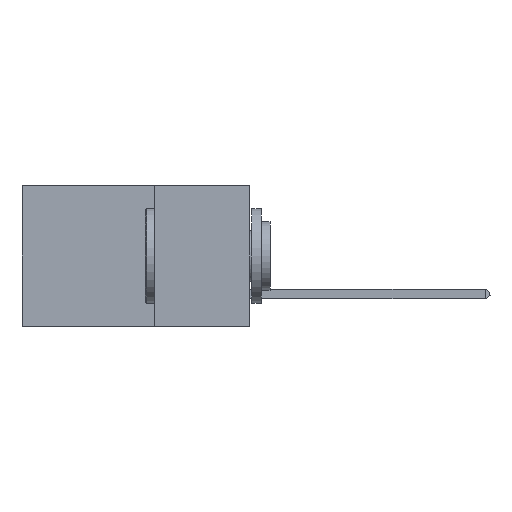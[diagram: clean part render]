
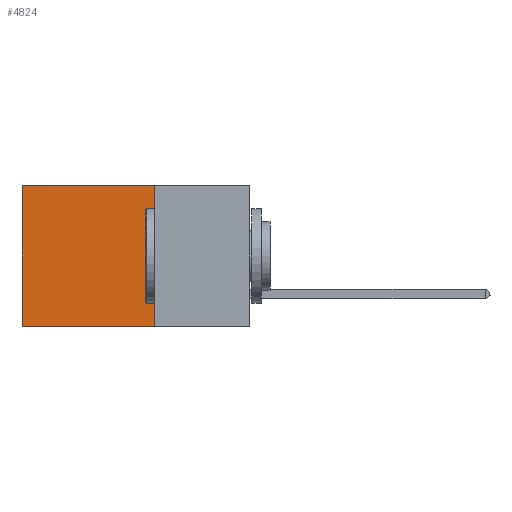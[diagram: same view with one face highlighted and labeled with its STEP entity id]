
A CAD part, left-side view. The second image highlights one B-rep face of the part: STEP entity #4824.
In plain terms, the highlighted planar face has unit normal (-1, 0, 0).
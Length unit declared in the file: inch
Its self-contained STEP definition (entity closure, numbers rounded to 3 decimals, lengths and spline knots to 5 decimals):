
#23 = DIRECTION ( 'NONE',  ( 0., 0., -1. ) ) ;
#262 = AXIS2_PLACEMENT_3D ( 'NONE', #18480, #22605, #1926 ) ;
#497 = CARTESIAN_POINT ( 'NONE',  ( 0.2875, 0.6, -0.37 ) ) ;
#527 = FACE_OUTER_BOUND ( 'NONE', #13912, .T. ) ;
#1441 = EDGE_CURVE ( 'NONE', #18868, #17375, #7194, .T. ) ;
#1840 = LINE ( 'NONE', #23936, #12132 ) ;
#1926 = DIRECTION ( 'NONE',  ( 0., 0., -1. ) ) ;
#2138 = CARTESIAN_POINT ( 'NONE',  ( 0.2875, 0.25, 0. ) ) ;
#3947 = VECTOR ( 'NONE', #8926, 39.37008 ) ;
#3976 = CARTESIAN_POINT ( 'NONE',  ( 0.2875, 0.6, 0. ) ) ;
#4824 = ADVANCED_FACE ( 'NONE', ( #527 ), #6069, .F. ) ;
#4943 = EDGE_CURVE ( 'NONE', #9010, #18868, #1840, .T. ) ;
#6069 = PLANE ( 'NONE',  #262 ) ;
#7194 = LINE ( 'NONE', #3976, #16951 ) ;
#7303 = VERTEX_POINT ( 'NONE', #14766 ) ;
#8643 = CARTESIAN_POINT ( 'NONE',  ( 0.2875, 0.6, 0. ) ) ;
#8926 = DIRECTION ( 'NONE',  ( 0., 1., 0. ) ) ;
#9010 = VERTEX_POINT ( 'NONE', #2138 ) ;
#10085 = ORIENTED_EDGE ( 'NONE', *, *, #1441, .T. ) ;
#10897 = CARTESIAN_POINT ( 'NONE',  ( 0.2875, 0.25, -0.37 ) ) ;
#12132 = VECTOR ( 'NONE', #19725, 39.37008 ) ;
#13284 = LINE ( 'NONE', #10897, #3947 ) ;
#13912 = EDGE_LOOP ( 'NONE', ( #10085, #21167, #14840, #20835 ) ) ;
#14743 = EDGE_CURVE ( 'NONE', #7303, #17375, #13284, .T. ) ;
#14766 = CARTESIAN_POINT ( 'NONE',  ( 0.2875, 0.25, -0.37 ) ) ;
#14840 = ORIENTED_EDGE ( 'NONE', *, *, #22328, .F. ) ;
#14953 = VECTOR ( 'NONE', #17335, 39.37008 ) ;
#16951 = VECTOR ( 'NONE', #23, 39.37008 ) ;
#17335 = DIRECTION ( 'NONE',  ( 0., 0., -1. ) ) ;
#17375 = VERTEX_POINT ( 'NONE', #497 ) ;
#18480 = CARTESIAN_POINT ( 'NONE',  ( 0.2875, 0.25, 0. ) ) ;
#18868 = VERTEX_POINT ( 'NONE', #8643 ) ;
#19327 = CARTESIAN_POINT ( 'NONE',  ( 0.2875, 0.25, 0. ) ) ;
#19725 = DIRECTION ( 'NONE',  ( 0., 1., 0. ) ) ;
#20469 = LINE ( 'NONE', #19327, #14953 ) ;
#20835 = ORIENTED_EDGE ( 'NONE', *, *, #4943, .T. ) ;
#21167 = ORIENTED_EDGE ( 'NONE', *, *, #14743, .F. ) ;
#22328 = EDGE_CURVE ( 'NONE', #9010, #7303, #20469, .T. ) ;
#22605 = DIRECTION ( 'NONE',  ( 1., 0., 0. ) ) ;
#23936 = CARTESIAN_POINT ( 'NONE',  ( 0.2875, 0.25, 0. ) ) ;
